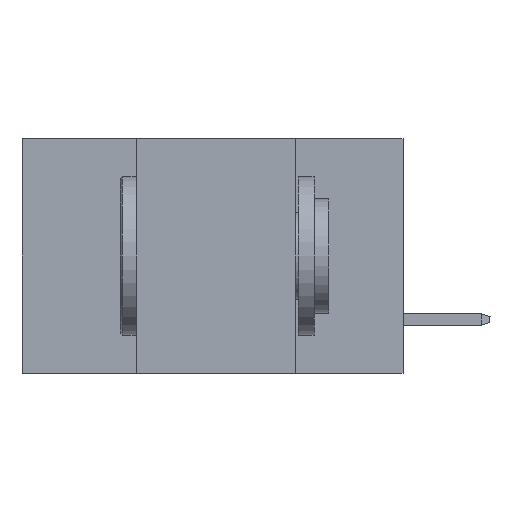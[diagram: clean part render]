
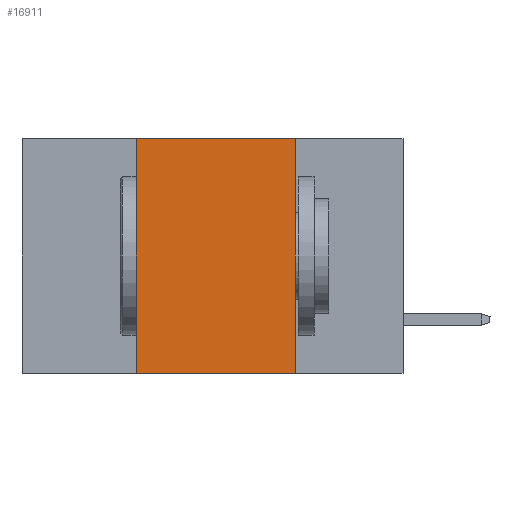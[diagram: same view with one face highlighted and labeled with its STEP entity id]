
A CAD part, left-side view. The second image highlights one B-rep face of the part: STEP entity #16911.
In plain terms, the highlighted planar face has unit normal (-1, 0, 0).
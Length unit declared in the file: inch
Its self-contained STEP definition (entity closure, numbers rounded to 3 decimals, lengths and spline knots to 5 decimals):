
#357 = EDGE_CURVE ( 'NONE', #27371, #9262, #27201, .T. ) ;
#1281 = DIRECTION ( 'NONE',  ( 0., 0., -1. ) ) ;
#3031 = DIRECTION ( 'NONE',  ( 0., 0., -1. ) ) ;
#4659 = ORIENTED_EDGE ( 'NONE', *, *, #357, .F. ) ;
#6833 = DIRECTION ( 'NONE',  ( 0., -1., 0. ) ) ;
#7002 = CARTESIAN_POINT ( 'NONE',  ( 0., 0.42, 0. ) ) ;
#8152 = AXIS2_PLACEMENT_3D ( 'NONE', #15718, #43414, #3031 ) ;
#8890 = VECTOR ( 'NONE', #34335, 39.37008 ) ;
#9256 = VERTEX_POINT ( 'NONE', #24200 ) ;
#9262 = VERTEX_POINT ( 'NONE', #7002 ) ;
#11376 = VERTEX_POINT ( 'NONE', #27584 ) ;
#11855 = ORIENTED_EDGE ( 'NONE', *, *, #25524, .T. ) ;
#13405 = DIRECTION ( 'NONE',  ( 0., 0., 1. ) ) ;
#14869 = CARTESIAN_POINT ( 'NONE',  ( 0., 0.17, 0. ) ) ;
#14922 = ORIENTED_EDGE ( 'NONE', *, *, #43358, .F. ) ;
#15718 = CARTESIAN_POINT ( 'NONE',  ( 0., 0.6, 0. ) ) ;
#16664 = LINE ( 'NONE', #40259, #8890 ) ;
#16911 = ADVANCED_FACE ( 'NONE', ( #39524 ), #32715, .F. ) ;
#17659 = LINE ( 'NONE', #24453, #33161 ) ;
#22387 = EDGE_LOOP ( 'NONE', ( #30635, #14922, #4659, #11855 ) ) ;
#24200 = CARTESIAN_POINT ( 'NONE',  ( 0., 0.17, -0.37 ) ) ;
#24453 = CARTESIAN_POINT ( 'NONE',  ( 0., 0.6, -0.37 ) ) ;
#24816 = EDGE_CURVE ( 'NONE', #11376, #9256, #25504, .T. ) ;
#25504 = LINE ( 'NONE', #14869, #31688 ) ;
#25524 = EDGE_CURVE ( 'NONE', #27371, #9256, #17659, .T. ) ;
#27201 = LINE ( 'NONE', #37877, #30658 ) ;
#27371 = VERTEX_POINT ( 'NONE', #36419 ) ;
#27584 = CARTESIAN_POINT ( 'NONE',  ( 0., 0.17, 0. ) ) ;
#30635 = ORIENTED_EDGE ( 'NONE', *, *, #24816, .F. ) ;
#30658 = VECTOR ( 'NONE', #13405, 39.37008 ) ;
#31688 = VECTOR ( 'NONE', #1281, 39.37008 ) ;
#32715 = PLANE ( 'NONE',  #8152 ) ;
#33161 = VECTOR ( 'NONE', #6833, 39.37008 ) ;
#34335 = DIRECTION ( 'NONE',  ( 0., -1., 0. ) ) ;
#36419 = CARTESIAN_POINT ( 'NONE',  ( 0., 0.42, -0.37 ) ) ;
#37877 = CARTESIAN_POINT ( 'NONE',  ( 0., 0.42, 0. ) ) ;
#39524 = FACE_OUTER_BOUND ( 'NONE', #22387, .T. ) ;
#40259 = CARTESIAN_POINT ( 'NONE',  ( 0., 0.6, 0. ) ) ;
#43358 = EDGE_CURVE ( 'NONE', #9262, #11376, #16664, .T. ) ;
#43414 = DIRECTION ( 'NONE',  ( 1., 0., 0. ) ) ;
